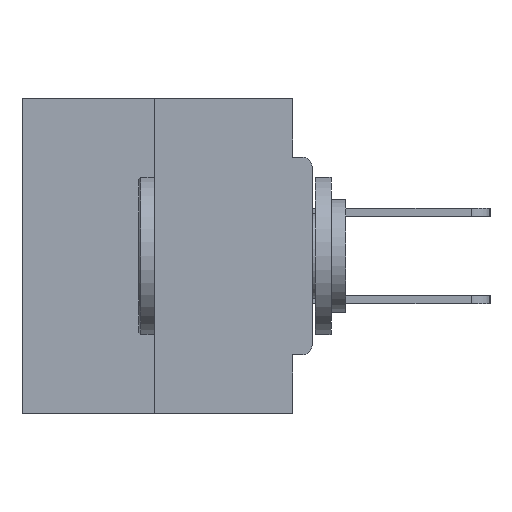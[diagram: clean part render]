
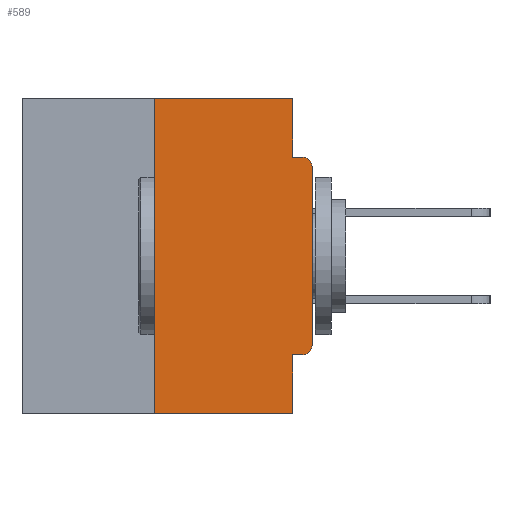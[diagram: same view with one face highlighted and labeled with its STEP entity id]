
A CAD part, left-side view. The second image highlights one B-rep face of the part: STEP entity #589.
In plain terms, the highlighted planar face has unit normal (-1, 0, 0).
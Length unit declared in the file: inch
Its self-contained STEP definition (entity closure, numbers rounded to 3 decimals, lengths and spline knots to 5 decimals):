
#134 = DIRECTION ( 'NONE',  ( -1., 0., 0. ) ) ;
#544 = CARTESIAN_POINT ( 'NONE',  ( 0., 0.031, -0.5 ) ) ;
#589 = ADVANCED_FACE ( 'NONE', ( #19665 ), #17494, .F. ) ;
#1039 = LINE ( 'NONE', #31930, #28582 ) ;
#1062 = CARTESIAN_POINT ( 'NONE',  ( 0., 0.46, 0. ) ) ;
#1400 = EDGE_CURVE ( 'NONE', #27664, #29682, #10872, .T. ) ;
#1427 = LINE ( 'NONE', #544, #27793 ) ;
#2088 = VERTEX_POINT ( 'NONE', #20984 ) ;
#2465 = CARTESIAN_POINT ( 'NONE',  ( 0., 0.46, -0.5 ) ) ;
#2681 = CARTESIAN_POINT ( 'NONE',  ( 0., 0.031, 0. ) ) ;
#4224 = ORIENTED_EDGE ( 'NONE', *, *, #17784, .F. ) ;
#4225 = LINE ( 'NONE', #2681, #14157 ) ;
#4862 = CARTESIAN_POINT ( 'NONE',  ( 0., 0.25, 0. ) ) ;
#4979 = DIRECTION ( 'NONE',  ( 0., 1., 0. ) ) ;
#5118 = ORIENTED_EDGE ( 'NONE', *, *, #27658, .F. ) ;
#6133 = VERTEX_POINT ( 'NONE', #15701 ) ;
#6490 = CIRCLE ( 'NONE', #14975, 0.015 ) ;
#6992 = DIRECTION ( 'NONE',  ( 1., 0., 0. ) ) ;
#7343 = EDGE_CURVE ( 'NONE', #27664, #13604, #32329, .T. ) ;
#8079 = CARTESIAN_POINT ( 'NONE',  ( 0., 0.015, -0.1085 ) ) ;
#8148 = CARTESIAN_POINT ( 'NONE',  ( 0., 0.25, 0. ) ) ;
#8981 = VERTEX_POINT ( 'NONE', #12522 ) ;
#9197 = ORIENTED_EDGE ( 'NONE', *, *, #30381, .F. ) ;
#9244 = EDGE_CURVE ( 'NONE', #21454, #28230, #4225, .T. ) ;
#9528 = DIRECTION ( 'NONE',  ( 0., 0., -1. ) ) ;
#10872 = LINE ( 'NONE', #2465, #30083 ) ;
#10900 = DIRECTION ( 'NONE',  ( 0., 0., -1. ) ) ;
#10917 = CARTESIAN_POINT ( 'NONE',  ( 0., 0., -0.0935 ) ) ;
#11013 = EDGE_CURVE ( 'NONE', #6133, #8981, #6490, .T. ) ;
#11512 = CIRCLE ( 'NONE', #16771, 0.015 ) ;
#12522 = CARTESIAN_POINT ( 'NONE',  ( 0., 0.015, -0.0935 ) ) ;
#13001 = DIRECTION ( 'NONE',  ( 0., 0., -1. ) ) ;
#13604 = VERTEX_POINT ( 'NONE', #4862 ) ;
#14045 = CARTESIAN_POINT ( 'NONE',  ( 0., 0.031, -0.0935 ) ) ;
#14157 = VECTOR ( 'NONE', #13001, 39.37008 ) ;
#14504 = CARTESIAN_POINT ( 'NONE',  ( 0., 0., -0.3915 ) ) ;
#14594 = LINE ( 'NONE', #1062, #24217 ) ;
#14653 = VECTOR ( 'NONE', #28240, 39.37008 ) ;
#14850 = DIRECTION ( 'NONE',  ( -1., 0., 0. ) ) ;
#14975 = AXIS2_PLACEMENT_3D ( 'NONE', #8079, #134, #25592 ) ;
#15701 = CARTESIAN_POINT ( 'NONE',  ( 0., 0., -0.1085 ) ) ;
#15824 = EDGE_CURVE ( 'NONE', #30682, #17208, #11512, .T. ) ;
#15865 = LINE ( 'NONE', #10917, #31945 ) ;
#16075 = CARTESIAN_POINT ( 'NONE',  ( 0., 0.031, 0. ) ) ;
#16771 = AXIS2_PLACEMENT_3D ( 'NONE', #28096, #14850, #20206 ) ;
#17208 = VERTEX_POINT ( 'NONE', #14504 ) ;
#17494 = PLANE ( 'NONE',  #20300 ) ;
#17784 = EDGE_CURVE ( 'NONE', #13604, #21454, #14594, .T. ) ;
#19228 = ORIENTED_EDGE ( 'NONE', *, *, #1400, .T. ) ;
#19533 = ORIENTED_EDGE ( 'NONE', *, *, #9244, .F. ) ;
#19665 = FACE_OUTER_BOUND ( 'NONE', #25338, .T. ) ;
#19924 = EDGE_CURVE ( 'NONE', #17208, #6133, #1039, .T. ) ;
#20206 = DIRECTION ( 'NONE',  ( 0., 0., -1. ) ) ;
#20237 = DIRECTION ( 'NONE',  ( 0., -1., 0. ) ) ;
#20300 = AXIS2_PLACEMENT_3D ( 'NONE', #29881, #6992, #9528 ) ;
#20984 = CARTESIAN_POINT ( 'NONE',  ( 0., 0.031, -0.4065 ) ) ;
#21454 = VERTEX_POINT ( 'NONE', #16075 ) ;
#21474 = DIRECTION ( 'NONE',  ( 0., 0., 1. ) ) ;
#21657 = DIRECTION ( 'NONE',  ( 0., -1., 0. ) ) ;
#23332 = ORIENTED_EDGE ( 'NONE', *, *, #7343, .F. ) ;
#23429 = DIRECTION ( 'NONE',  ( 0., -1., 0. ) ) ;
#24217 = VECTOR ( 'NONE', #21657, 39.37008 ) ;
#24345 = ORIENTED_EDGE ( 'NONE', *, *, #19924, .T. ) ;
#24750 = CARTESIAN_POINT ( 'NONE',  ( 0., 0.015, -0.4065 ) ) ;
#25228 = EDGE_CURVE ( 'NONE', #30682, #2088, #30104, .T. ) ;
#25338 = EDGE_LOOP ( 'NONE', ( #4224, #23332, #19228, #9197, #28283, #26474, #24345, #26857, #5118, #19533 ) ) ;
#25592 = DIRECTION ( 'NONE',  ( 0., 0., -1. ) ) ;
#26474 = ORIENTED_EDGE ( 'NONE', *, *, #15824, .T. ) ;
#26857 = ORIENTED_EDGE ( 'NONE', *, *, #11013, .T. ) ;
#27658 = EDGE_CURVE ( 'NONE', #28230, #8981, #15865, .T. ) ;
#27664 = VERTEX_POINT ( 'NONE', #31280 ) ;
#27793 = VECTOR ( 'NONE', #10900, 39.37008 ) ;
#28096 = CARTESIAN_POINT ( 'NONE',  ( 0., 0.015, -0.3915 ) ) ;
#28230 = VERTEX_POINT ( 'NONE', #14045 ) ;
#28240 = DIRECTION ( 'NONE',  ( 0., 0., 1. ) ) ;
#28283 = ORIENTED_EDGE ( 'NONE', *, *, #25228, .F. ) ;
#28491 = VECTOR ( 'NONE', #4979, 39.37008 ) ;
#28582 = VECTOR ( 'NONE', #21474, 39.37008 ) ;
#29682 = VERTEX_POINT ( 'NONE', #30252 ) ;
#29881 = CARTESIAN_POINT ( 'NONE',  ( 0., 0.46, 0. ) ) ;
#30083 = VECTOR ( 'NONE', #20237, 39.37008 ) ;
#30104 = LINE ( 'NONE', #33117, #28491 ) ;
#30252 = CARTESIAN_POINT ( 'NONE',  ( 0., 0.031, -0.5 ) ) ;
#30381 = EDGE_CURVE ( 'NONE', #2088, #29682, #1427, .T. ) ;
#30682 = VERTEX_POINT ( 'NONE', #24750 ) ;
#31280 = CARTESIAN_POINT ( 'NONE',  ( 0., 0.25, -0.5 ) ) ;
#31930 = CARTESIAN_POINT ( 'NONE',  ( 0., 0., 0. ) ) ;
#31945 = VECTOR ( 'NONE', #23429, 39.37008 ) ;
#32329 = LINE ( 'NONE', #8148, #14653 ) ;
#33117 = CARTESIAN_POINT ( 'NONE',  ( 0., 0., -0.4065 ) ) ;
